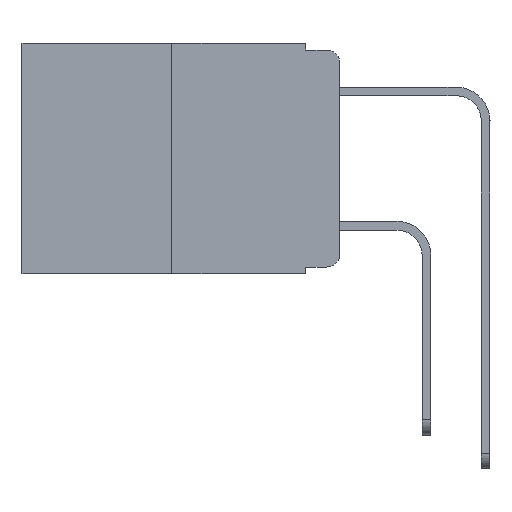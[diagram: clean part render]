
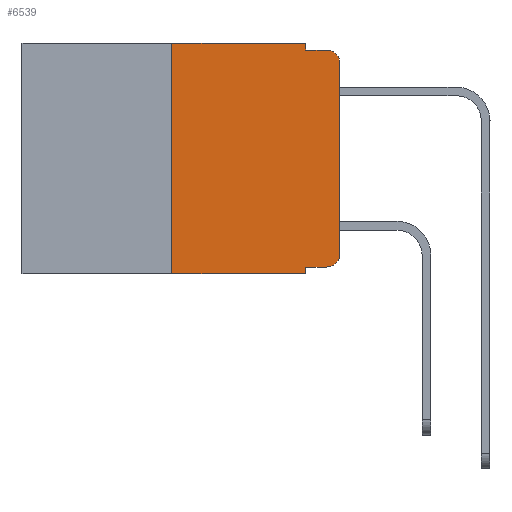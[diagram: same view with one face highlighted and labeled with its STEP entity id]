
A CAD part, left-side view. The second image highlights one B-rep face of the part: STEP entity #6539.
In plain terms, the highlighted planar face has unit normal (-1, 0, 0).
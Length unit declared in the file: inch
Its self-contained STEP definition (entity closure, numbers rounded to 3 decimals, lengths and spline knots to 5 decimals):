
#64 = DIRECTION ( 'NONE',  ( -1., 0., 0. ) ) ;
#123 = VERTEX_POINT ( 'NONE', #4895 ) ;
#324 = EDGE_CURVE ( 'NONE', #1861, #10924, #5070, .T. ) ;
#521 = EDGE_CURVE ( 'NONE', #3141, #13489, #5580, .T. ) ;
#598 = AXIS2_PLACEMENT_3D ( 'NONE', #7013, #64, #8110 ) ;
#759 = VERTEX_POINT ( 'NONE', #5790 ) ;
#849 = CARTESIAN_POINT ( 'NONE',  ( 0., 0.051, -0.333 ) ) ;
#869 = EDGE_LOOP ( 'NONE', ( #1953, #4313, #5544, #7987, #1753, #10204, #4259, #1038, #4075, #7180 ) ) ;
#912 = VECTOR ( 'NONE', #5377, 39.37008 ) ;
#1029 = VECTOR ( 'NONE', #7591, 39.37008 ) ;
#1038 = ORIENTED_EDGE ( 'NONE', *, *, #14507, .F. ) ;
#1199 = CARTESIAN_POINT ( 'NONE',  ( 0., 0.473, 0. ) ) ;
#1753 = ORIENTED_EDGE ( 'NONE', *, *, #9604, .F. ) ;
#1837 = LINE ( 'NONE', #4590, #5275 ) ;
#1861 = VERTEX_POINT ( 'NONE', #11006 ) ;
#1953 = ORIENTED_EDGE ( 'NONE', *, *, #3776, .T. ) ;
#1958 = CARTESIAN_POINT ( 'NONE',  ( 0., 0., 0. ) ) ;
#2122 = VECTOR ( 'NONE', #4689, 39.37008 ) ;
#3102 = LINE ( 'NONE', #11555, #3457 ) ;
#3141 = VERTEX_POINT ( 'NONE', #5542 ) ;
#3457 = VECTOR ( 'NONE', #4975, 39.37008 ) ;
#3514 = VERTEX_POINT ( 'NONE', #5056 ) ;
#3590 = VERTEX_POINT ( 'NONE', #4083 ) ;
#3776 = EDGE_CURVE ( 'NONE', #759, #3141, #4241, .T. ) ;
#4075 = ORIENTED_EDGE ( 'NONE', *, *, #11666, .T. ) ;
#4083 = CARTESIAN_POINT ( 'NONE',  ( 0., 0.02, -0.333 ) ) ;
#4228 = VECTOR ( 'NONE', #6727, 39.37008 ) ;
#4241 = LINE ( 'NONE', #1958, #1029 ) ;
#4259 = ORIENTED_EDGE ( 'NONE', *, *, #324, .T. ) ;
#4313 = ORIENTED_EDGE ( 'NONE', *, *, #521, .T. ) ;
#4462 = CARTESIAN_POINT ( 'NONE',  ( 0., 0.051, -0.343 ) ) ;
#4590 = CARTESIAN_POINT ( 'NONE',  ( 0., 0.051, -0.333 ) ) ;
#4689 = DIRECTION ( 'NONE',  ( 0., 0., 1. ) ) ;
#4787 = PLANE ( 'NONE',  #10438 ) ;
#4895 = CARTESIAN_POINT ( 'NONE',  ( 0., 0.25, 0. ) ) ;
#4975 = DIRECTION ( 'NONE',  ( 0., 0., -1. ) ) ;
#5056 = CARTESIAN_POINT ( 'NONE',  ( 0., 0.051, -0.01 ) ) ;
#5070 = LINE ( 'NONE', #5953, #13761 ) ;
#5187 = LINE ( 'NONE', #9047, #2122 ) ;
#5275 = VECTOR ( 'NONE', #11127, 39.37008 ) ;
#5377 = DIRECTION ( 'NONE',  ( 0., -1., 0. ) ) ;
#5463 = DIRECTION ( 'NONE',  ( -1., 0., 0. ) ) ;
#5542 = CARTESIAN_POINT ( 'NONE',  ( 0., 0., -0.03 ) ) ;
#5544 = ORIENTED_EDGE ( 'NONE', *, *, #12863, .F. ) ;
#5580 = CIRCLE ( 'NONE', #12352, 0.02 ) ;
#5790 = CARTESIAN_POINT ( 'NONE',  ( 0., 0., -0.313 ) ) ;
#5890 = DIRECTION ( 'NONE',  ( 1., 0., 0. ) ) ;
#5953 = CARTESIAN_POINT ( 'NONE',  ( 0., 0.473, -0.343 ) ) ;
#6050 = CIRCLE ( 'NONE', #598, 0.02 ) ;
#6185 = VERTEX_POINT ( 'NONE', #12967 ) ;
#6484 = DIRECTION ( 'NONE',  ( 0., -1., 0. ) ) ;
#6539 = ADVANCED_FACE ( 'NONE', ( #10676 ), #4787, .F. ) ;
#6727 = DIRECTION ( 'NONE',  ( 0., -1., 0. ) ) ;
#7002 = EDGE_CURVE ( 'NONE', #1861, #123, #5187, .T. ) ;
#7013 = CARTESIAN_POINT ( 'NONE',  ( 0., 0.02, -0.313 ) ) ;
#7037 = DIRECTION ( 'NONE',  ( 0., 0., -1. ) ) ;
#7180 = ORIENTED_EDGE ( 'NONE', *, *, #8755, .T. ) ;
#7591 = DIRECTION ( 'NONE',  ( 0., 0., 1. ) ) ;
#7987 = ORIENTED_EDGE ( 'NONE', *, *, #9944, .F. ) ;
#8110 = DIRECTION ( 'NONE',  ( 0., 0., -1. ) ) ;
#8130 = CARTESIAN_POINT ( 'NONE',  ( 0., 0.051, 0. ) ) ;
#8755 = EDGE_CURVE ( 'NONE', #3590, #759, #6050, .T. ) ;
#8757 = VECTOR ( 'NONE', #7037, 39.37008 ) ;
#8932 = CARTESIAN_POINT ( 'NONE',  ( 0., 0.051, -0.01 ) ) ;
#9047 = CARTESIAN_POINT ( 'NONE',  ( 0., 0.25, 0. ) ) ;
#9149 = VERTEX_POINT ( 'NONE', #849 ) ;
#9604 = EDGE_CURVE ( 'NONE', #123, #6185, #12852, .T. ) ;
#9635 = CARTESIAN_POINT ( 'NONE',  ( 0., 0.02, -0.01 ) ) ;
#9680 = CARTESIAN_POINT ( 'NONE',  ( 0., 0.473, 0. ) ) ;
#9944 = EDGE_CURVE ( 'NONE', #6185, #3514, #11649, .T. ) ;
#10204 = ORIENTED_EDGE ( 'NONE', *, *, #7002, .F. ) ;
#10438 = AXIS2_PLACEMENT_3D ( 'NONE', #1199, #5890, #13515 ) ;
#10676 = FACE_OUTER_BOUND ( 'NONE', #869, .T. ) ;
#10924 = VERTEX_POINT ( 'NONE', #4462 ) ;
#11006 = CARTESIAN_POINT ( 'NONE',  ( 0., 0.25, -0.343 ) ) ;
#11127 = DIRECTION ( 'NONE',  ( 0., -1., 0. ) ) ;
#11555 = CARTESIAN_POINT ( 'NONE',  ( 0., 0.051, 0. ) ) ;
#11649 = LINE ( 'NONE', #8130, #8757 ) ;
#11666 = EDGE_CURVE ( 'NONE', #9149, #3590, #1837, .T. ) ;
#12352 = AXIS2_PLACEMENT_3D ( 'NONE', #12591, #5463, #13408 ) ;
#12591 = CARTESIAN_POINT ( 'NONE',  ( 0., 0.02, -0.03 ) ) ;
#12610 = LINE ( 'NONE', #8932, #4228 ) ;
#12852 = LINE ( 'NONE', #9680, #912 ) ;
#12863 = EDGE_CURVE ( 'NONE', #3514, #13489, #12610, .T. ) ;
#12967 = CARTESIAN_POINT ( 'NONE',  ( 0., 0.051, 0. ) ) ;
#13408 = DIRECTION ( 'NONE',  ( 0., 0., -1. ) ) ;
#13489 = VERTEX_POINT ( 'NONE', #9635 ) ;
#13515 = DIRECTION ( 'NONE',  ( 0., 0., -1. ) ) ;
#13761 = VECTOR ( 'NONE', #6484, 39.37008 ) ;
#14507 = EDGE_CURVE ( 'NONE', #9149, #10924, #3102, .T. ) ;
